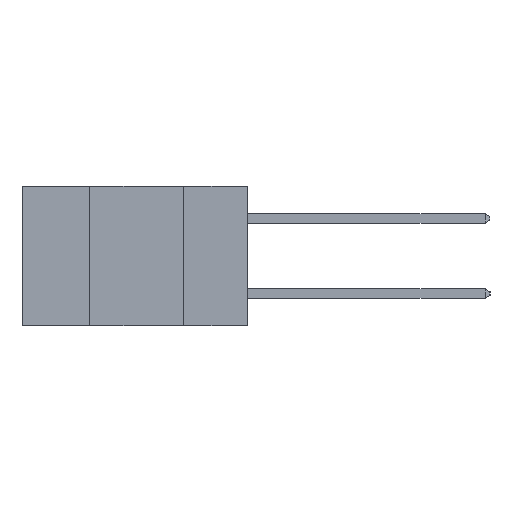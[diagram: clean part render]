
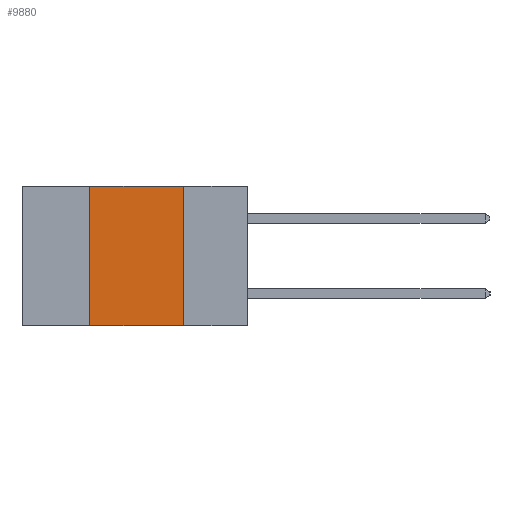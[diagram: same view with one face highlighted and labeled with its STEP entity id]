
A CAD part, left-side view. The second image highlights one B-rep face of the part: STEP entity #9880.
In plain terms, the highlighted planar face has unit normal (-1, 0, 0).
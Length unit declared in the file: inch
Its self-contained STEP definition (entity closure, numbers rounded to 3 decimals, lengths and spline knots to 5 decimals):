
#18 = LINE ( 'NONE', #8818, #10887 ) ;
#316 = EDGE_CURVE ( 'NONE', #16053, #7928, #10515, .T. ) ;
#317 = DIRECTION ( 'NONE',  ( 0., 0., 1. ) ) ;
#456 = CARTESIAN_POINT ( 'NONE',  ( 0., 0.42, 0. ) ) ;
#650 = DIRECTION ( 'NONE',  ( 0., -1., 0. ) ) ;
#1647 = DIRECTION ( 'NONE',  ( 1., 0., 0. ) ) ;
#1882 = EDGE_LOOP ( 'NONE', ( #2761, #13610, #15951, #3608 ) ) ;
#2460 = VERTEX_POINT ( 'NONE', #456 ) ;
#2494 = DIRECTION ( 'NONE',  ( 0., -1., 0. ) ) ;
#2761 = ORIENTED_EDGE ( 'NONE', *, *, #316, .F. ) ;
#3608 = ORIENTED_EDGE ( 'NONE', *, *, #14993, .T. ) ;
#3978 = CARTESIAN_POINT ( 'NONE',  ( 0., 0.17, -0.37 ) ) ;
#4466 = VECTOR ( 'NONE', #317, 39.37008 ) ;
#5344 = DIRECTION ( 'NONE',  ( 0., 0., -1. ) ) ;
#7109 = CARTESIAN_POINT ( 'NONE',  ( 0., 0.42, -0.37 ) ) ;
#7349 = LINE ( 'NONE', #8834, #14149 ) ;
#7360 = VERTEX_POINT ( 'NONE', #13912 ) ;
#7902 = CARTESIAN_POINT ( 'NONE',  ( 0., 0.17, 0. ) ) ;
#7928 = VERTEX_POINT ( 'NONE', #15031 ) ;
#8818 = CARTESIAN_POINT ( 'NONE',  ( 0., 0.6, -0.37 ) ) ;
#8834 = CARTESIAN_POINT ( 'NONE',  ( 0., 0.6, 0. ) ) ;
#8945 = EDGE_CURVE ( 'NONE', #2460, #16053, #7349, .T. ) ;
#9813 = PLANE ( 'NONE',  #9843 ) ;
#9843 = AXIS2_PLACEMENT_3D ( 'NONE', #15202, #1647, #11154 ) ;
#9880 = ADVANCED_FACE ( 'NONE', ( #17510 ), #9813, .F. ) ;
#10515 = LINE ( 'NONE', #3978, #17270 ) ;
#10887 = VECTOR ( 'NONE', #650, 39.37008 ) ;
#11154 = DIRECTION ( 'NONE',  ( 0., 0., -1. ) ) ;
#13610 = ORIENTED_EDGE ( 'NONE', *, *, #8945, .F. ) ;
#13912 = CARTESIAN_POINT ( 'NONE',  ( 0., 0.42, -0.37 ) ) ;
#14149 = VECTOR ( 'NONE', #2494, 39.37008 ) ;
#14904 = LINE ( 'NONE', #7109, #4466 ) ;
#14993 = EDGE_CURVE ( 'NONE', #7360, #7928, #18, .T. ) ;
#15031 = CARTESIAN_POINT ( 'NONE',  ( 0., 0.17, -0.37 ) ) ;
#15202 = CARTESIAN_POINT ( 'NONE',  ( 0., 0.6, 0. ) ) ;
#15787 = EDGE_CURVE ( 'NONE', #7360, #2460, #14904, .T. ) ;
#15951 = ORIENTED_EDGE ( 'NONE', *, *, #15787, .F. ) ;
#16053 = VERTEX_POINT ( 'NONE', #7902 ) ;
#17270 = VECTOR ( 'NONE', #5344, 39.37008 ) ;
#17510 = FACE_OUTER_BOUND ( 'NONE', #1882, .T. ) ;
